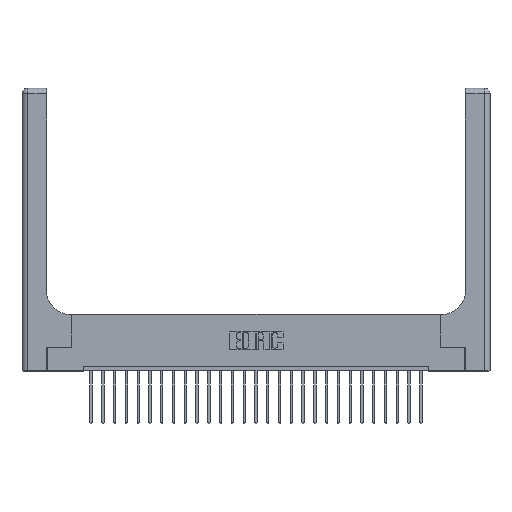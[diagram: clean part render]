
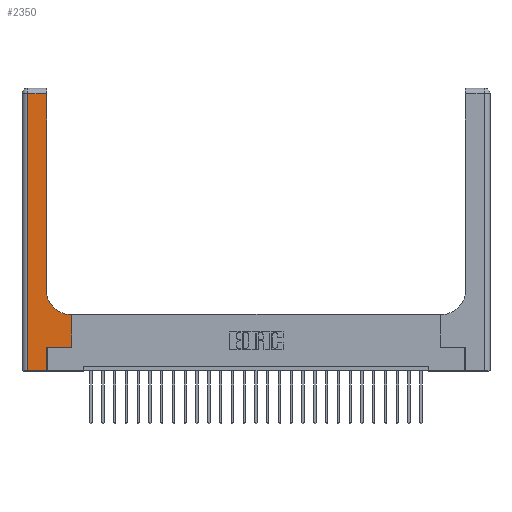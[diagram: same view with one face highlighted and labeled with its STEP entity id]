
A CAD part, top view. The second image highlights one B-rep face of the part: STEP entity #2350.
In plain terms, the highlighted planar face has unit normal (0, 0, 1).
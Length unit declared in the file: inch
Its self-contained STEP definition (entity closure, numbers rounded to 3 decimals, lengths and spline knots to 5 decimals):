
#787 = LINE ( 'NONE', #21233, #20712 ) ;
#1221 = DIRECTION ( 'NONE',  ( 0., 1., 0. ) ) ;
#1538 = VERTEX_POINT ( 'NONE', #12601 ) ;
#1618 = VERTEX_POINT ( 'NONE', #18907 ) ;
#1784 = VECTOR ( 'NONE', #12361, 39.37008 ) ;
#2216 = ORIENTED_EDGE ( 'NONE', *, *, #24484, .T. ) ;
#2350 = ADVANCED_FACE ( 'NONE', ( #8633 ), #23172, .F. ) ;
#2388 = EDGE_CURVE ( 'NONE', #6329, #1618, #787, .T. ) ;
#2775 = VECTOR ( 'NONE', #22465, 39.37008 ) ;
#2867 = ORIENTED_EDGE ( 'NONE', *, *, #6224, .T. ) ;
#3554 = ORIENTED_EDGE ( 'NONE', *, *, #6296, .T. ) ;
#3621 = DIRECTION ( 'NONE',  ( 0., 0., -1. ) ) ;
#3874 = DIRECTION ( 'NONE',  ( -1., 0., 0. ) ) ;
#4070 = LINE ( 'NONE', #22394, #8015 ) ;
#4175 = VERTEX_POINT ( 'NONE', #22550 ) ;
#4412 = CARTESIAN_POINT ( 'NONE',  ( 0.06, 0., 0.37 ) ) ;
#4587 = LINE ( 'NONE', #11413, #23256 ) ;
#6161 = CARTESIAN_POINT ( 'NONE',  ( 0.26, 2.94, 0.37 ) ) ;
#6224 = EDGE_CURVE ( 'NONE', #1618, #24420, #15389, .T. ) ;
#6296 = EDGE_CURVE ( 'NONE', #24420, #4175, #20926, .T. ) ;
#6329 = VERTEX_POINT ( 'NONE', #4412 ) ;
#7438 = CARTESIAN_POINT ( 'NONE',  ( 0.06, 2.94, 0.37 ) ) ;
#7981 = VERTEX_POINT ( 'NONE', #24635 ) ;
#8015 = VECTOR ( 'NONE', #1221, 39.37008 ) ;
#8195 = LINE ( 'NONE', #14930, #17206 ) ;
#8577 = ORIENTED_EDGE ( 'NONE', *, *, #24353, .T. ) ;
#8633 = FACE_OUTER_BOUND ( 'NONE', #16351, .T. ) ;
#10450 = CARTESIAN_POINT ( 'NONE',  ( 0.51, 0.85, 0.37 ) ) ;
#11361 = ORIENTED_EDGE ( 'NONE', *, *, #15242, .T. ) ;
#11413 = CARTESIAN_POINT ( 'NONE',  ( 0., 2.94, 0.37 ) ) ;
#11526 = CIRCLE ( 'NONE', #15201, 0.25 ) ;
#11973 = AXIS2_PLACEMENT_3D ( 'NONE', #15435, #3621, #3874 ) ;
#12114 = LINE ( 'NONE', #17471, #18732 ) ;
#12232 = EDGE_CURVE ( 'NONE', #4175, #1538, #4070, .T. ) ;
#12361 = DIRECTION ( 'NONE',  ( 0., 1., 0. ) ) ;
#12442 = CARTESIAN_POINT ( 'NONE',  ( 0.265, 0., 0.37 ) ) ;
#12601 = CARTESIAN_POINT ( 'NONE',  ( 0.528, 0.6, 0.37 ) ) ;
#12874 = VERTEX_POINT ( 'NONE', #7438 ) ;
#13928 = CARTESIAN_POINT ( 'NONE',  ( 0.265, 0.25, 0.37 ) ) ;
#14000 = VERTEX_POINT ( 'NONE', #6161 ) ;
#14214 = ORIENTED_EDGE ( 'NONE', *, *, #15923, .T. ) ;
#14576 = DIRECTION ( 'NONE',  ( 0., 0., -1. ) ) ;
#14930 = CARTESIAN_POINT ( 'NONE',  ( 0.26, 3., 0.37 ) ) ;
#14948 = ORIENTED_EDGE ( 'NONE', *, *, #24863, .T. ) ;
#15201 = AXIS2_PLACEMENT_3D ( 'NONE', #10450, #14576, #23923 ) ;
#15242 = EDGE_CURVE ( 'NONE', #12874, #6329, #22992, .T. ) ;
#15301 = DIRECTION ( 'NONE',  ( -1., 0., 0. ) ) ;
#15389 = LINE ( 'NONE', #12442, #1784 ) ;
#15435 = CARTESIAN_POINT ( 'NONE',  ( 0., 3., 0.37 ) ) ;
#15872 = DIRECTION ( 'NONE',  ( 1., 0., 0. ) ) ;
#15923 = EDGE_CURVE ( 'NONE', #1538, #7981, #12114, .T. ) ;
#16351 = EDGE_LOOP ( 'NONE', ( #14948, #2216, #11361, #22437, #2867, #3554, #16982, #14214, #8577 ) ) ;
#16982 = ORIENTED_EDGE ( 'NONE', *, *, #12232, .T. ) ;
#17139 = CARTESIAN_POINT ( 'NONE',  ( 0.265, 0.25, 0.37 ) ) ;
#17206 = VECTOR ( 'NONE', #24426, 39.37008 ) ;
#17471 = CARTESIAN_POINT ( 'NONE',  ( 0.26, 0.6, 0.37 ) ) ;
#18732 = VECTOR ( 'NONE', #23298, 39.37008 ) ;
#18907 = CARTESIAN_POINT ( 'NONE',  ( 0.265, 0., 0.37 ) ) ;
#20529 = CARTESIAN_POINT ( 'NONE',  ( 0.06, 3., 0.37 ) ) ;
#20639 = VECTOR ( 'NONE', #15872, 39.37008 ) ;
#20712 = VECTOR ( 'NONE', #22932, 39.37008 ) ;
#20926 = LINE ( 'NONE', #13928, #20639 ) ;
#21074 = CARTESIAN_POINT ( 'NONE',  ( 0.26, 0.85, 0.37 ) ) ;
#21233 = CARTESIAN_POINT ( 'NONE',  ( 0., 0., 0.37 ) ) ;
#22394 = CARTESIAN_POINT ( 'NONE',  ( 0.528, 0.25, 0.37 ) ) ;
#22437 = ORIENTED_EDGE ( 'NONE', *, *, #2388, .T. ) ;
#22465 = DIRECTION ( 'NONE',  ( 0., -1., 0. ) ) ;
#22550 = CARTESIAN_POINT ( 'NONE',  ( 0.528, 0.25, 0.37 ) ) ;
#22932 = DIRECTION ( 'NONE',  ( 1., 0., 0. ) ) ;
#22992 = LINE ( 'NONE', #20529, #2775 ) ;
#23172 = PLANE ( 'NONE',  #11973 ) ;
#23256 = VECTOR ( 'NONE', #15301, 39.37008 ) ;
#23298 = DIRECTION ( 'NONE',  ( -1., 0., 0. ) ) ;
#23890 = VERTEX_POINT ( 'NONE', #21074 ) ;
#23923 = DIRECTION ( 'NONE',  ( 1., 0., 0. ) ) ;
#24353 = EDGE_CURVE ( 'NONE', #7981, #23890, #11526, .T. ) ;
#24420 = VERTEX_POINT ( 'NONE', #17139 ) ;
#24426 = DIRECTION ( 'NONE',  ( 0., 1., 0. ) ) ;
#24484 = EDGE_CURVE ( 'NONE', #14000, #12874, #4587, .T. ) ;
#24635 = CARTESIAN_POINT ( 'NONE',  ( 0.51, 0.6, 0.37 ) ) ;
#24863 = EDGE_CURVE ( 'NONE', #23890, #14000, #8195, .T. ) ;
